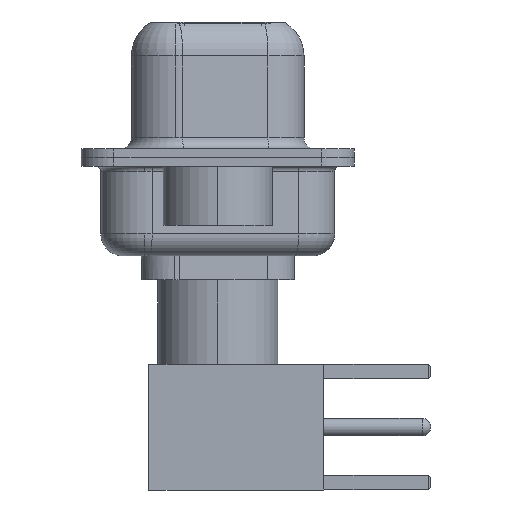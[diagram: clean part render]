
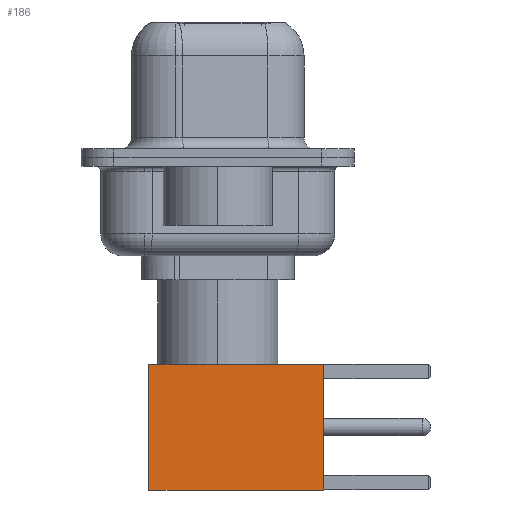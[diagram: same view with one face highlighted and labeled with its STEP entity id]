
A CAD part, left-side view. The second image highlights one B-rep face of the part: STEP entity #186.
In plain terms, the highlighted face is planar.
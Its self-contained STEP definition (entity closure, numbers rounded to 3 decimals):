
#186 = ADVANCED_FACE ( 'NONE', ( #15329 ), #6779, .T. ) ;
#1582 = DIRECTION ( 'NONE',  ( 0., 1., 0. ) ) ;
#2032 = LINE ( 'NONE', #5631, #2792 ) ;
#2165 = CARTESIAN_POINT ( 'NONE',  ( 2.875, 2.875, 8. ) ) ;
#2792 = VECTOR ( 'NONE', #14501, 1000. ) ;
#3320 = EDGE_CURVE ( 'NONE', #12874, #12582, #4766, .T. ) ;
#3912 = EDGE_CURVE ( 'NONE', #14723, #5161, #10192, .T. ) ;
#4588 = VECTOR ( 'NONE', #9731, 1000. ) ;
#4766 = LINE ( 'NONE', #14789, #4588 ) ;
#4838 = AXIS2_PLACEMENT_3D ( 'NONE', #7751, #1582, #14050 ) ;
#5161 = VERTEX_POINT ( 'NONE', #5369 ) ;
#5369 = CARTESIAN_POINT ( 'NONE',  ( 2.875, 2.875, 0. ) ) ;
#5631 = CARTESIAN_POINT ( 'NONE',  ( 0., 2.875, 0. ) ) ;
#6779 = PLANE ( 'NONE',  #4838 ) ;
#7733 = CARTESIAN_POINT ( 'NONE',  ( -2.875, 2.875, 0. ) ) ;
#7741 = CARTESIAN_POINT ( 'NONE',  ( 2.875, 2.875, 0. ) ) ;
#7751 = CARTESIAN_POINT ( 'NONE',  ( 2.875, 2.875, 0. ) ) ;
#8282 = VECTOR ( 'NONE', #12368, 1000. ) ;
#8647 = VECTOR ( 'NONE', #10366, 1000. ) ;
#9596 = CARTESIAN_POINT ( 'NONE',  ( -2.875, 2.875, 8. ) ) ;
#9731 = DIRECTION ( 'NONE',  ( 0., 0., -1. ) ) ;
#10171 = CARTESIAN_POINT ( 'NONE',  ( 0., 2.875, 8. ) ) ;
#10192 = LINE ( 'NONE', #7741, #8647 ) ;
#10366 = DIRECTION ( 'NONE',  ( 0., 0., -1. ) ) ;
#11384 = LINE ( 'NONE', #10171, #8282 ) ;
#11707 = ORIENTED_EDGE ( 'NONE', *, *, #3320, .F. ) ;
#11880 = EDGE_LOOP ( 'NONE', ( #12486, #13330, #11707, #15457 ) ) ;
#12368 = DIRECTION ( 'NONE',  ( -1., 0., 0. ) ) ;
#12486 = ORIENTED_EDGE ( 'NONE', *, *, #3912, .T. ) ;
#12582 = VERTEX_POINT ( 'NONE', #7733 ) ;
#12874 = VERTEX_POINT ( 'NONE', #9596 ) ;
#12915 = EDGE_CURVE ( 'NONE', #5161, #12582, #2032, .T. ) ;
#13330 = ORIENTED_EDGE ( 'NONE', *, *, #12915, .T. ) ;
#14050 = DIRECTION ( 'NONE',  ( 0., 0., 1. ) ) ;
#14501 = DIRECTION ( 'NONE',  ( -1., 0., 0. ) ) ;
#14723 = VERTEX_POINT ( 'NONE', #2165 ) ;
#14789 = CARTESIAN_POINT ( 'NONE',  ( -2.875, 2.875, 0. ) ) ;
#15329 = FACE_OUTER_BOUND ( 'NONE', #11880, .T. ) ;
#15457 = ORIENTED_EDGE ( 'NONE', *, *, #15581, .F. ) ;
#15581 = EDGE_CURVE ( 'NONE', #14723, #12874, #11384, .T. ) ;
